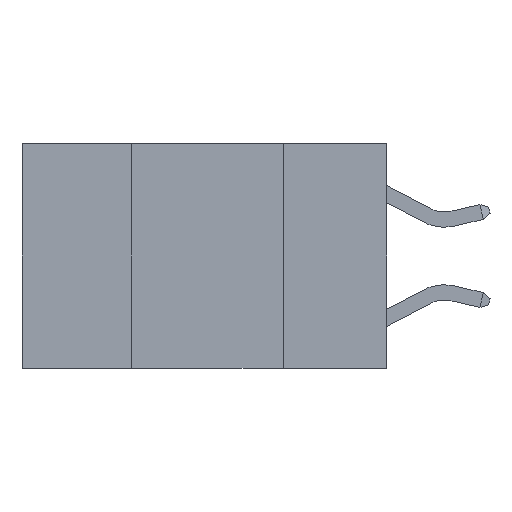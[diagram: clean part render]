
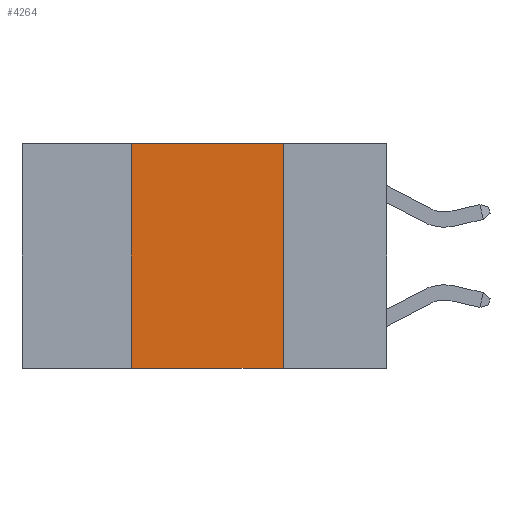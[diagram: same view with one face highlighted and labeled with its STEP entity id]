
A CAD part, left-side view. The second image highlights one B-rep face of the part: STEP entity #4264.
In plain terms, the highlighted planar face has unit normal (-1, 0, 0).
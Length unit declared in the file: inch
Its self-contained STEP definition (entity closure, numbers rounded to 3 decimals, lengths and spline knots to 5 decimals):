
#501 = EDGE_LOOP ( 'NONE', ( #9652, #16587, #14452, #15960 ) ) ;
#583 = VECTOR ( 'NONE', #10015, 39.37008 ) ;
#1145 = LINE ( 'NONE', #20504, #583 ) ;
#2814 = CARTESIAN_POINT ( 'NONE',  ( 0., 0.42, 0. ) ) ;
#4264 = ADVANCED_FACE ( 'NONE', ( #4944 ), #19141, .F. ) ;
#4516 = LINE ( 'NONE', #18588, #11095 ) ;
#4944 = FACE_OUTER_BOUND ( 'NONE', #501, .T. ) ;
#6532 = CARTESIAN_POINT ( 'NONE',  ( 0., 0.42, -0.37 ) ) ;
#6703 = CARTESIAN_POINT ( 'NONE',  ( 0., 0.6, 0. ) ) ;
#6935 = EDGE_CURVE ( 'NONE', #21186, #13883, #1145, .T. ) ;
#7590 = DIRECTION ( 'NONE',  ( 0., 0., 1. ) ) ;
#8613 = DIRECTION ( 'NONE',  ( 1., 0., 0. ) ) ;
#9652 = ORIENTED_EDGE ( 'NONE', *, *, #14102, .F. ) ;
#9684 = VECTOR ( 'NONE', #14938, 39.37008 ) ;
#9838 = CARTESIAN_POINT ( 'NONE',  ( 0., 0.17, -0.37 ) ) ;
#10015 = DIRECTION ( 'NONE',  ( 0., -1., 0. ) ) ;
#11095 = VECTOR ( 'NONE', #13187, 39.37008 ) ;
#13187 = DIRECTION ( 'NONE',  ( 0., -1., 0. ) ) ;
#13216 = LINE ( 'NONE', #2814, #20266 ) ;
#13883 = VERTEX_POINT ( 'NONE', #18122 ) ;
#14102 = EDGE_CURVE ( 'NONE', #13883, #20445, #18580, .T. ) ;
#14452 = ORIENTED_EDGE ( 'NONE', *, *, #19993, .F. ) ;
#14938 = DIRECTION ( 'NONE',  ( 0., 0., -1. ) ) ;
#14973 = VERTEX_POINT ( 'NONE', #6532 ) ;
#15156 = CARTESIAN_POINT ( 'NONE',  ( 0., 0.42, 0. ) ) ;
#15182 = CARTESIAN_POINT ( 'NONE',  ( 0., 0.17, 0. ) ) ;
#15446 = AXIS2_PLACEMENT_3D ( 'NONE', #6703, #8613, #20964 ) ;
#15960 = ORIENTED_EDGE ( 'NONE', *, *, #21973, .T. ) ;
#16587 = ORIENTED_EDGE ( 'NONE', *, *, #6935, .F. ) ;
#18122 = CARTESIAN_POINT ( 'NONE',  ( 0., 0.17, 0. ) ) ;
#18580 = LINE ( 'NONE', #15182, #9684 ) ;
#18588 = CARTESIAN_POINT ( 'NONE',  ( 0., 0.6, -0.37 ) ) ;
#19141 = PLANE ( 'NONE',  #15446 ) ;
#19993 = EDGE_CURVE ( 'NONE', #14973, #21186, #13216, .T. ) ;
#20266 = VECTOR ( 'NONE', #7590, 39.37008 ) ;
#20445 = VERTEX_POINT ( 'NONE', #9838 ) ;
#20504 = CARTESIAN_POINT ( 'NONE',  ( 0., 0.6, 0. ) ) ;
#20964 = DIRECTION ( 'NONE',  ( 0., 0., -1. ) ) ;
#21186 = VERTEX_POINT ( 'NONE', #15156 ) ;
#21973 = EDGE_CURVE ( 'NONE', #14973, #20445, #4516, .T. ) ;
